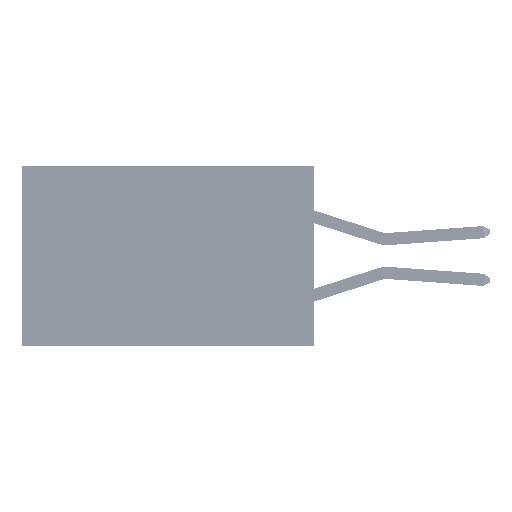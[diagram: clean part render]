
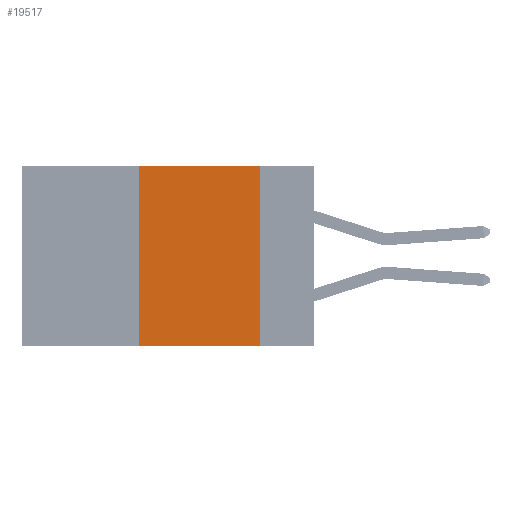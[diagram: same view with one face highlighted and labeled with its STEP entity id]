
A CAD part, left-side view. The second image highlights one B-rep face of the part: STEP entity #19517.
In plain terms, the highlighted planar face has unit normal (-1, 0, 0).
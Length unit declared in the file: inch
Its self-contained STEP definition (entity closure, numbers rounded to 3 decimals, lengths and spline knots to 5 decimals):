
#40 = CARTESIAN_POINT ( 'NONE',  ( 0., 0.6, -0.37 ) ) ;
#109 = CARTESIAN_POINT ( 'NONE',  ( 0., 0.11, 0. ) ) ;
#1277 = VECTOR ( 'NONE', #14401, 39.37008 ) ;
#1401 = CARTESIAN_POINT ( 'NONE',  ( 0., 0.6, 0. ) ) ;
#2561 = DIRECTION ( 'NONE',  ( 0., 0., 1. ) ) ;
#4067 = DIRECTION ( 'NONE',  ( 0., -1., 0. ) ) ;
#4213 = VERTEX_POINT ( 'NONE', #109 ) ;
#4298 = ORIENTED_EDGE ( 'NONE', *, *, #32717, .T. ) ;
#6137 = EDGE_LOOP ( 'NONE', ( #41238, #15467, #34408, #4298 ) ) ;
#6627 = DIRECTION ( 'NONE',  ( 1., 0., 0. ) ) ;
#10239 = LINE ( 'NONE', #39059, #51647 ) ;
#10995 = VECTOR ( 'NONE', #4067, 39.37008 ) ;
#11950 = LINE ( 'NONE', #38481, #1277 ) ;
#14401 = DIRECTION ( 'NONE',  ( 0., 0., -1. ) ) ;
#14505 = PLANE ( 'NONE',  #34291 ) ;
#15467 = ORIENTED_EDGE ( 'NONE', *, *, #42465, .F. ) ;
#15703 = CARTESIAN_POINT ( 'NONE',  ( 0., 0.36, -0.37 ) ) ;
#15911 = CARTESIAN_POINT ( 'NONE',  ( 0., 0.11, -0.37 ) ) ;
#18569 = CARTESIAN_POINT ( 'NONE',  ( 0., 0.6, 0. ) ) ;
#19517 = ADVANCED_FACE ( 'NONE', ( #41191 ), #14505, .F. ) ;
#32326 = LINE ( 'NONE', #40, #10995 ) ;
#32717 = EDGE_CURVE ( 'NONE', #33395, #48468, #32326, .T. ) ;
#33334 = LINE ( 'NONE', #1401, #42158 ) ;
#33395 = VERTEX_POINT ( 'NONE', #15703 ) ;
#33835 = CARTESIAN_POINT ( 'NONE',  ( 0., 0.36, 0. ) ) ;
#34291 = AXIS2_PLACEMENT_3D ( 'NONE', #18569, #6627, #38771 ) ;
#34408 = ORIENTED_EDGE ( 'NONE', *, *, #41336, .F. ) ;
#36515 = EDGE_CURVE ( 'NONE', #4213, #48468, #11950, .T. ) ;
#38481 = CARTESIAN_POINT ( 'NONE',  ( 0., 0.11, 0. ) ) ;
#38771 = DIRECTION ( 'NONE',  ( 0., 0., -1. ) ) ;
#39059 = CARTESIAN_POINT ( 'NONE',  ( 0., 0.36, 0. ) ) ;
#41191 = FACE_OUTER_BOUND ( 'NONE', #6137, .T. ) ;
#41238 = ORIENTED_EDGE ( 'NONE', *, *, #36515, .F. ) ;
#41336 = EDGE_CURVE ( 'NONE', #33395, #48639, #10239, .T. ) ;
#42158 = VECTOR ( 'NONE', #45770, 39.37008 ) ;
#42465 = EDGE_CURVE ( 'NONE', #48639, #4213, #33334, .T. ) ;
#45770 = DIRECTION ( 'NONE',  ( 0., -1., 0. ) ) ;
#48468 = VERTEX_POINT ( 'NONE', #15911 ) ;
#48639 = VERTEX_POINT ( 'NONE', #33835 ) ;
#51647 = VECTOR ( 'NONE', #2561, 39.37008 ) ;
